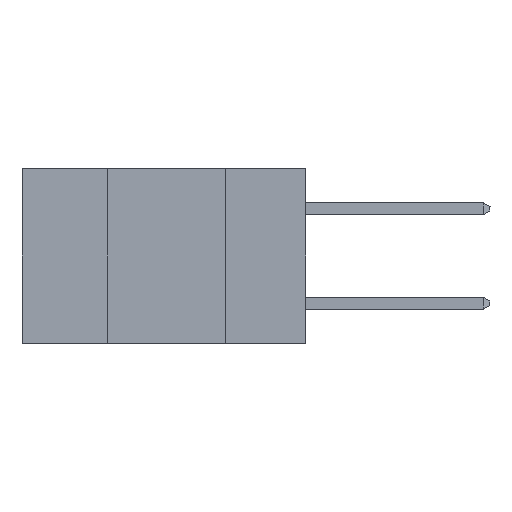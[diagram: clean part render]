
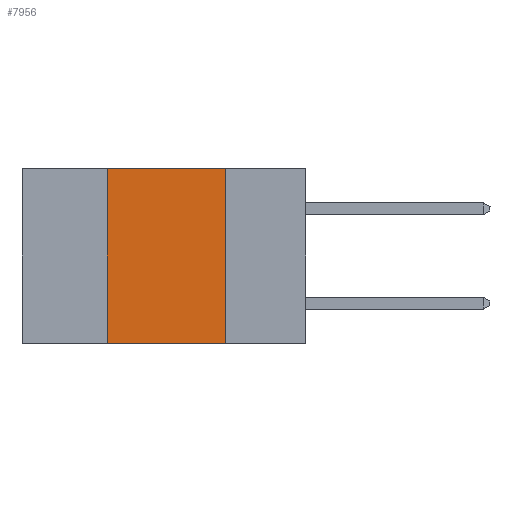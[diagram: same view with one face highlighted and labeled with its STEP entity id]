
A CAD part, left-side view. The second image highlights one B-rep face of the part: STEP entity #7956.
In plain terms, the highlighted planar face has unit normal (-1, 0, 0).
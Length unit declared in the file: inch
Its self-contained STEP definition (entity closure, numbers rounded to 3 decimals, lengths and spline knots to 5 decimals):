
#524 = EDGE_CURVE ( 'NONE', #5013, #6043, #24778, .T. ) ;
#570 = VECTOR ( 'NONE', #14274, 39.37008 ) ;
#1381 = ORIENTED_EDGE ( 'NONE', *, *, #10217, .F. ) ;
#1812 = DIRECTION ( 'NONE',  ( 0., -1., 0. ) ) ;
#1919 = VERTEX_POINT ( 'NONE', #4886 ) ;
#3234 = DIRECTION ( 'NONE',  ( 0., 0., -1. ) ) ;
#4886 = CARTESIAN_POINT ( 'NONE',  ( 0., 0.42, -0.37 ) ) ;
#5013 = VERTEX_POINT ( 'NONE', #13649 ) ;
#6043 = VERTEX_POINT ( 'NONE', #8462 ) ;
#6075 = LINE ( 'NONE', #24535, #570 ) ;
#7956 = ADVANCED_FACE ( 'NONE', ( #12341 ), #13511, .F. ) ;
#8462 = CARTESIAN_POINT ( 'NONE',  ( 0., 0.17, -0.37 ) ) ;
#8660 = EDGE_CURVE ( 'NONE', #1919, #15063, #22281, .T. ) ;
#10173 = LINE ( 'NONE', #26497, #20492 ) ;
#10217 = EDGE_CURVE ( 'NONE', #15063, #5013, #6075, .T. ) ;
#10439 = ORIENTED_EDGE ( 'NONE', *, *, #21120, .T. ) ;
#11428 = ORIENTED_EDGE ( 'NONE', *, *, #524, .F. ) ;
#11746 = ORIENTED_EDGE ( 'NONE', *, *, #8660, .F. ) ;
#11881 = DIRECTION ( 'NONE',  ( 0., 0., 1. ) ) ;
#12341 = FACE_OUTER_BOUND ( 'NONE', #16886, .T. ) ;
#13175 = VECTOR ( 'NONE', #19918, 39.37008 ) ;
#13511 = PLANE ( 'NONE',  #18460 ) ;
#13570 = CARTESIAN_POINT ( 'NONE',  ( 0., 0.17, -0.37 ) ) ;
#13649 = CARTESIAN_POINT ( 'NONE',  ( 0., 0.17, 0. ) ) ;
#14274 = DIRECTION ( 'NONE',  ( 0., -1., 0. ) ) ;
#15063 = VERTEX_POINT ( 'NONE', #16833 ) ;
#15546 = DIRECTION ( 'NONE',  ( 1., 0., 0. ) ) ;
#16833 = CARTESIAN_POINT ( 'NONE',  ( 0., 0.42, 0. ) ) ;
#16886 = EDGE_LOOP ( 'NONE', ( #11428, #1381, #11746, #10439 ) ) ;
#18460 = AXIS2_PLACEMENT_3D ( 'NONE', #23755, #15546, #3234 ) ;
#19918 = DIRECTION ( 'NONE',  ( 0., 0., -1. ) ) ;
#20073 = CARTESIAN_POINT ( 'NONE',  ( 0., 0.42, -0.37 ) ) ;
#20492 = VECTOR ( 'NONE', #1812, 39.37008 ) ;
#21120 = EDGE_CURVE ( 'NONE', #1919, #6043, #10173, .T. ) ;
#21636 = VECTOR ( 'NONE', #11881, 39.37008 ) ;
#22281 = LINE ( 'NONE', #20073, #21636 ) ;
#23755 = CARTESIAN_POINT ( 'NONE',  ( 0., 0.6, 0. ) ) ;
#24535 = CARTESIAN_POINT ( 'NONE',  ( 0., 0.6, 0. ) ) ;
#24778 = LINE ( 'NONE', #13570, #13175 ) ;
#26497 = CARTESIAN_POINT ( 'NONE',  ( 0., 0.6, -0.37 ) ) ;
